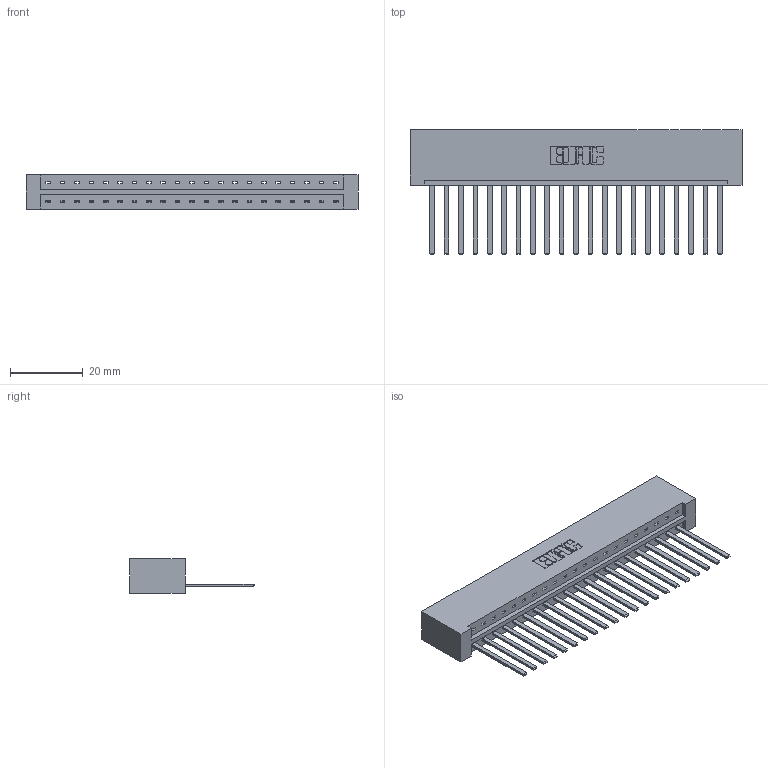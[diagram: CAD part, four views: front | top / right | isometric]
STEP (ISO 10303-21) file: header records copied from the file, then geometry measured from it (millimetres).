
FILE_DESCRIPTION (( 'STEP AP203' ), '1' );
FILE_NAME ('333-021-544-101.STEP', '2018-08-02T01:16:55', ( '' ), ( '' ), 'SwSTEP 2.0', 'SolidWorks 2016', '' );
FILE_SCHEMA (( 'CONFIG_CONTROL_DESIGN' ));
Length unit declared in the file: inch
Products named in the file (3): 333 Part_Lugless; 345-292-001_345-293-144; 333-021-544-101
Assembly tree (22 placements, depth 2):
  333-021-544-101
    333 Part_Lugless
    345-292-001_345-293-144  x21
Bounding box: 91.47 x 34.3 x 9.4 mm (x, y, z)
Volume: 9879.4 mm3; surface area: 11299.2 mm2
Topology: 22 solids, 22 shells, 1198 faces, 3605 edges, 2374 vertices
Faces by surface type: plane 864, cylinder 334
Entity records: 15093 total; most frequent: CARTESIAN_POINT 2613, ORIENTED_EDGE 2570, DIRECTION 2235, EDGE_CURVE 1285, VECTOR 1169, LINE 1169, VERTEX_POINT 854, AXIS2_PLACEMENT_3D 533
